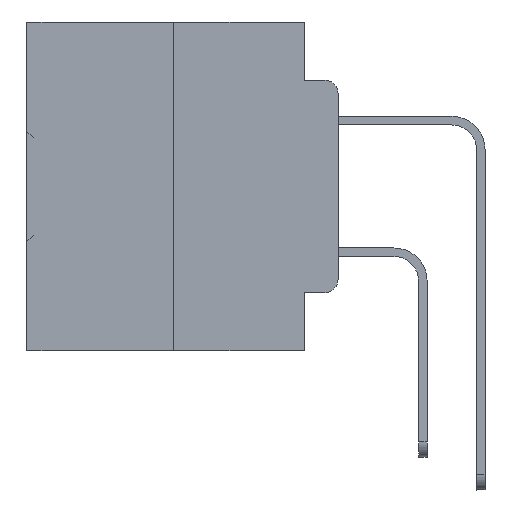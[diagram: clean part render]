
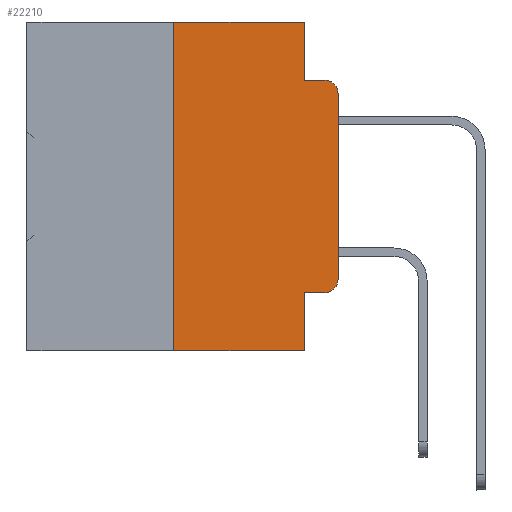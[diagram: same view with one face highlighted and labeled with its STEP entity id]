
A CAD part, left-side view. The second image highlights one B-rep face of the part: STEP entity #22210.
In plain terms, the highlighted planar face has unit normal (-1, 0, 0).
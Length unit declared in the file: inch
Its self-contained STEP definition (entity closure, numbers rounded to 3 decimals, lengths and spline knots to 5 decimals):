
#61 = DIRECTION ( 'NONE',  ( 1., 0., 0. ) ) ;
#1197 = DIRECTION ( 'NONE',  ( 0., 0., -1. ) ) ;
#1633 = EDGE_CURVE ( 'NONE', #7354, #3812, #31099, .T. ) ;
#2327 = VERTEX_POINT ( 'NONE', #20218 ) ;
#3528 = EDGE_CURVE ( 'NONE', #6784, #13408, #8680, .T. ) ;
#3812 = VERTEX_POINT ( 'NONE', #15789 ) ;
#4694 = CARTESIAN_POINT ( 'NONE',  ( 0., 0.25, 0. ) ) ;
#5132 = VERTEX_POINT ( 'NONE', #22017 ) ;
#6638 = DIRECTION ( 'NONE',  ( 0., 0., -1. ) ) ;
#6784 = VERTEX_POINT ( 'NONE', #38345 ) ;
#6933 = CARTESIAN_POINT ( 'NONE',  ( 0., 0.25, 0. ) ) ;
#6955 = VECTOR ( 'NONE', #25792, 39.37008 ) ;
#7354 = VERTEX_POINT ( 'NONE', #34080 ) ;
#7491 = ORIENTED_EDGE ( 'NONE', *, *, #24532, .F. ) ;
#7548 = DIRECTION ( 'NONE',  ( 0., 0., 1. ) ) ;
#7617 = VECTOR ( 'NONE', #12618, 39.37008 ) ;
#7813 = VERTEX_POINT ( 'NONE', #30315 ) ;
#8026 = CARTESIAN_POINT ( 'NONE',  ( 0., 0.02, -0.3915 ) ) ;
#8421 = CARTESIAN_POINT ( 'NONE',  ( 0., 0.25, -0.5 ) ) ;
#8680 = LINE ( 'NONE', #33936, #23700 ) ;
#10474 = VECTOR ( 'NONE', #6638, 39.37008 ) ;
#10724 = LINE ( 'NONE', #17684, #17739 ) ;
#11118 = DIRECTION ( 'NONE',  ( 0., 0., -1. ) ) ;
#12109 = ORIENTED_EDGE ( 'NONE', *, *, #16518, .F. ) ;
#12618 = DIRECTION ( 'NONE',  ( 0., -1., 0. ) ) ;
#13408 = VERTEX_POINT ( 'NONE', #22061 ) ;
#13742 = AXIS2_PLACEMENT_3D ( 'NONE', #8026, #28965, #11118 ) ;
#14275 = VECTOR ( 'NONE', #7548, 39.37008 ) ;
#14668 = DIRECTION ( 'NONE',  ( 0., 0., -1. ) ) ;
#14973 = CARTESIAN_POINT ( 'NONE',  ( 0., 0., -0.3915 ) ) ;
#15024 = LINE ( 'NONE', #4694, #6955 ) ;
#15489 = EDGE_CURVE ( 'NONE', #22136, #7354, #22255, .T. ) ;
#15575 = LINE ( 'NONE', #23983, #38193 ) ;
#15789 = CARTESIAN_POINT ( 'NONE',  ( 0., 0.02, -0.0885 ) ) ;
#16299 = VERTEX_POINT ( 'NONE', #8421 ) ;
#16518 = EDGE_CURVE ( 'NONE', #7813, #2327, #25443, .T. ) ;
#17027 = EDGE_CURVE ( 'NONE', #33908, #7813, #15575, .T. ) ;
#17378 = CARTESIAN_POINT ( 'NONE',  ( 0., 0.051, -0.0885 ) ) ;
#17684 = CARTESIAN_POINT ( 'NONE',  ( 0., 0.051, 0. ) ) ;
#17739 = VECTOR ( 'NONE', #14668, 39.37008 ) ;
#18099 = DIRECTION ( 'NONE',  ( 0., -1., 0. ) ) ;
#18459 = EDGE_LOOP ( 'NONE', ( #23725, #32963, #26575, #12109, #27165, #21586, #29936, #7491, #24923, #26345 ) ) ;
#19240 = FACE_OUTER_BOUND ( 'NONE', #18459, .T. ) ;
#19519 = CARTESIAN_POINT ( 'NONE',  ( 0., 0., 0. ) ) ;
#19984 = AXIS2_PLACEMENT_3D ( 'NONE', #34397, #20188, #1197 ) ;
#20001 = DIRECTION ( 'NONE',  ( 0., -1., 0. ) ) ;
#20188 = DIRECTION ( 'NONE',  ( -1., 0., 0. ) ) ;
#20218 = CARTESIAN_POINT ( 'NONE',  ( 0., 0.051, -0.0885 ) ) ;
#21370 = DIRECTION ( 'NONE',  ( 0., 0., -1. ) ) ;
#21586 = ORIENTED_EDGE ( 'NONE', *, *, #22539, .F. ) ;
#22017 = CARTESIAN_POINT ( 'NONE',  ( 0., 0.051, -0.5 ) ) ;
#22061 = CARTESIAN_POINT ( 'NONE',  ( 0., 0.02, -0.4115 ) ) ;
#22136 = VERTEX_POINT ( 'NONE', #14973 ) ;
#22210 = ADVANCED_FACE ( 'NONE', ( #19240 ), #36052, .F. ) ;
#22255 = LINE ( 'NONE', #19519, #14275 ) ;
#22539 = EDGE_CURVE ( 'NONE', #16299, #33908, #15024, .T. ) ;
#23279 = EDGE_CURVE ( 'NONE', #2327, #3812, #35346, .T. ) ;
#23700 = VECTOR ( 'NONE', #20001, 39.37008 ) ;
#23725 = ORIENTED_EDGE ( 'NONE', *, *, #15489, .T. ) ;
#23983 = CARTESIAN_POINT ( 'NONE',  ( 0., 0.473, 0. ) ) ;
#24532 = EDGE_CURVE ( 'NONE', #6784, #5132, #10724, .T. ) ;
#24685 = CARTESIAN_POINT ( 'NONE',  ( 0., 0.051, 0. ) ) ;
#24923 = ORIENTED_EDGE ( 'NONE', *, *, #3528, .T. ) ;
#25443 = LINE ( 'NONE', #24685, #10474 ) ;
#25792 = DIRECTION ( 'NONE',  ( 0., 0., 1. ) ) ;
#26345 = ORIENTED_EDGE ( 'NONE', *, *, #32424, .T. ) ;
#26575 = ORIENTED_EDGE ( 'NONE', *, *, #23279, .F. ) ;
#27165 = ORIENTED_EDGE ( 'NONE', *, *, #17027, .F. ) ;
#27586 = VECTOR ( 'NONE', #29333, 39.37008 ) ;
#28965 = DIRECTION ( 'NONE',  ( -1., 0., 0. ) ) ;
#29333 = DIRECTION ( 'NONE',  ( 0., -1., 0. ) ) ;
#29936 = ORIENTED_EDGE ( 'NONE', *, *, #33433, .T. ) ;
#30172 = CARTESIAN_POINT ( 'NONE',  ( 0., 0.473, 0. ) ) ;
#30315 = CARTESIAN_POINT ( 'NONE',  ( 0., 0.051, 0. ) ) ;
#31099 = CIRCLE ( 'NONE', #19984, 0.02 ) ;
#31704 = AXIS2_PLACEMENT_3D ( 'NONE', #30172, #61, #21370 ) ;
#32424 = EDGE_CURVE ( 'NONE', #13408, #22136, #32840, .T. ) ;
#32840 = CIRCLE ( 'NONE', #13742, 0.02 ) ;
#32963 = ORIENTED_EDGE ( 'NONE', *, *, #1633, .T. ) ;
#33385 = CARTESIAN_POINT ( 'NONE',  ( 0., 0.473, -0.5 ) ) ;
#33433 = EDGE_CURVE ( 'NONE', #16299, #5132, #37372, .T. ) ;
#33908 = VERTEX_POINT ( 'NONE', #6933 ) ;
#33936 = CARTESIAN_POINT ( 'NONE',  ( 0., 0.051, -0.4115 ) ) ;
#34080 = CARTESIAN_POINT ( 'NONE',  ( 0., 0., -0.1085 ) ) ;
#34397 = CARTESIAN_POINT ( 'NONE',  ( 0., 0.02, -0.1085 ) ) ;
#35346 = LINE ( 'NONE', #17378, #27586 ) ;
#36052 = PLANE ( 'NONE',  #31704 ) ;
#37372 = LINE ( 'NONE', #33385, #7617 ) ;
#38193 = VECTOR ( 'NONE', #18099, 39.37008 ) ;
#38345 = CARTESIAN_POINT ( 'NONE',  ( 0., 0.051, -0.4115 ) ) ;
